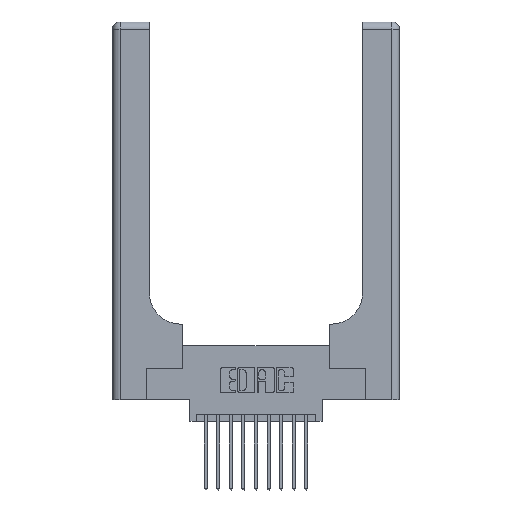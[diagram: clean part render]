
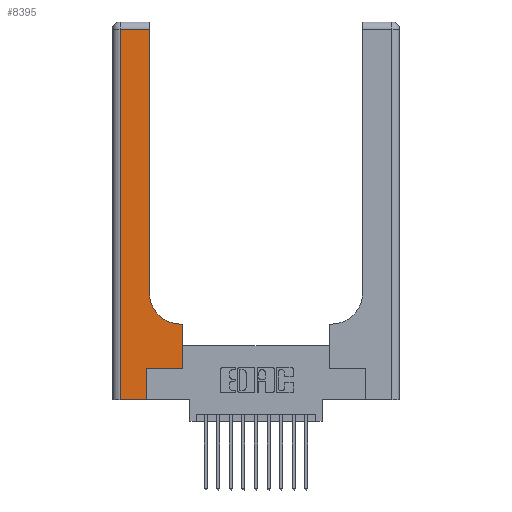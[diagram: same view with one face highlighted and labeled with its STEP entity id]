
A CAD part, top view. The second image highlights one B-rep face of the part: STEP entity #8395.
In plain terms, the highlighted planar face has unit normal (0, 0, 1).
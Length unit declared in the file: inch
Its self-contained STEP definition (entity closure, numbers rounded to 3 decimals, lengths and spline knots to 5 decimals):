
#37 = DIRECTION ( 'NONE',  ( 1., 0., 0. ) ) ;
#104 = VECTOR ( 'NONE', #10363, 39.37008 ) ;
#362 = LINE ( 'NONE', #11340, #13898 ) ;
#521 = LINE ( 'NONE', #15537, #104 ) ;
#1140 = CARTESIAN_POINT ( 'NONE',  ( 0.5585, 0.25, 0.37 ) ) ;
#1219 = VERTEX_POINT ( 'NONE', #10721 ) ;
#1307 = VERTEX_POINT ( 'NONE', #4497 ) ;
#1602 = LINE ( 'NONE', #8688, #14653 ) ;
#1817 = CIRCLE ( 'NONE', #6236, 0.25 ) ;
#2074 = CARTESIAN_POINT ( 'NONE',  ( 0.269, 0., 0.37 ) ) ;
#2140 = ORIENTED_EDGE ( 'NONE', *, *, #8368, .T. ) ;
#2536 = EDGE_CURVE ( 'NONE', #1307, #12621, #1602, .T. ) ;
#2644 = LINE ( 'NONE', #6530, #9198 ) ;
#2702 = VERTEX_POINT ( 'NONE', #1140 ) ;
#2889 = EDGE_CURVE ( 'NONE', #15873, #1219, #1817, .T. ) ;
#3220 = EDGE_CURVE ( 'NONE', #14287, #15873, #13449, .T. ) ;
#3399 = EDGE_CURVE ( 'NONE', #1219, #1307, #521, .T. ) ;
#3471 = DIRECTION ( 'NONE',  ( -1., 0., 0. ) ) ;
#3485 = FACE_OUTER_BOUND ( 'NONE', #14809, .T. ) ;
#4211 = ORIENTED_EDGE ( 'NONE', *, *, #3399, .T. ) ;
#4497 = CARTESIAN_POINT ( 'NONE',  ( 0.2915, 2.94, 0.37 ) ) ;
#4805 = DIRECTION ( 'NONE',  ( 0., 1., 0. ) ) ;
#4854 = DIRECTION ( 'NONE',  ( -1., 0., 0. ) ) ;
#4859 = PLANE ( 'NONE',  #8008 ) ;
#4885 = ORIENTED_EDGE ( 'NONE', *, *, #3220, .T. ) ;
#5260 = ORIENTED_EDGE ( 'NONE', *, *, #5963, .T. ) ;
#5262 = CARTESIAN_POINT ( 'NONE',  ( 0.269, 0.25, 0.37 ) ) ;
#5963 = EDGE_CURVE ( 'NONE', #10393, #14970, #16134, .T. ) ;
#6160 = DIRECTION ( 'NONE',  ( -1., 0., 0. ) ) ;
#6236 = AXIS2_PLACEMENT_3D ( 'NONE', #14668, #6862, #15933 ) ;
#6530 = CARTESIAN_POINT ( 'NONE',  ( 0.269, 0.25, 0.37 ) ) ;
#6651 = EDGE_CURVE ( 'NONE', #9863, #10393, #13339, .T. ) ;
#6862 = DIRECTION ( 'NONE',  ( 0., 0., -1. ) ) ;
#6885 = DIRECTION ( 'NONE',  ( 1., 0., 0. ) ) ;
#7643 = VECTOR ( 'NONE', #6885, 39.37008 ) ;
#7901 = DIRECTION ( 'NONE',  ( 0., -1., 0. ) ) ;
#8008 = AXIS2_PLACEMENT_3D ( 'NONE', #12649, #13997, #6160 ) ;
#8184 = CARTESIAN_POINT ( 'NONE',  ( 0.06, 2.94, 0.37 ) ) ;
#8368 = EDGE_CURVE ( 'NONE', #2702, #14287, #362, .T. ) ;
#8395 = ADVANCED_FACE ( 'NONE', ( #3485 ), #4859, .F. ) ;
#8688 = CARTESIAN_POINT ( 'NONE',  ( 0., 2.94, 0.37 ) ) ;
#9198 = VECTOR ( 'NONE', #37, 39.37008 ) ;
#9303 = VECTOR ( 'NONE', #13883, 39.37008 ) ;
#9345 = CARTESIAN_POINT ( 'NONE',  ( 0.269, 0., 0.37 ) ) ;
#9600 = VECTOR ( 'NONE', #4854, 39.37008 ) ;
#9863 = VERTEX_POINT ( 'NONE', #10834 ) ;
#10087 = CARTESIAN_POINT ( 'NONE',  ( 0.2915, 0.6, 0.37 ) ) ;
#10334 = EDGE_CURVE ( 'NONE', #12621, #9863, #14892, .T. ) ;
#10363 = DIRECTION ( 'NONE',  ( 0., 1., 0. ) ) ;
#10393 = VERTEX_POINT ( 'NONE', #9345 ) ;
#10721 = CARTESIAN_POINT ( 'NONE',  ( 0.2915, 0.85, 0.37 ) ) ;
#10834 = CARTESIAN_POINT ( 'NONE',  ( 0.06, 0., 0.37 ) ) ;
#10854 = ORIENTED_EDGE ( 'NONE', *, *, #10334, .T. ) ;
#11127 = EDGE_CURVE ( 'NONE', #14970, #2702, #2644, .T. ) ;
#11340 = CARTESIAN_POINT ( 'NONE',  ( 0.5585, 0.25, 0.37 ) ) ;
#12313 = ORIENTED_EDGE ( 'NONE', *, *, #6651, .T. ) ;
#12621 = VERTEX_POINT ( 'NONE', #8184 ) ;
#12649 = CARTESIAN_POINT ( 'NONE',  ( 0., 3., 0.37 ) ) ;
#12746 = CARTESIAN_POINT ( 'NONE',  ( 0.5415, 0.6, 0.37 ) ) ;
#13014 = CARTESIAN_POINT ( 'NONE',  ( 0.5585, 0.6, 0.37 ) ) ;
#13339 = LINE ( 'NONE', #14693, #7643 ) ;
#13449 = LINE ( 'NONE', #10087, #9600 ) ;
#13556 = ORIENTED_EDGE ( 'NONE', *, *, #2889, .T. ) ;
#13883 = DIRECTION ( 'NONE',  ( 0., 1., 0. ) ) ;
#13898 = VECTOR ( 'NONE', #4805, 39.37008 ) ;
#13997 = DIRECTION ( 'NONE',  ( 0., 0., -1. ) ) ;
#14095 = VECTOR ( 'NONE', #7901, 39.37008 ) ;
#14287 = VERTEX_POINT ( 'NONE', #13014 ) ;
#14653 = VECTOR ( 'NONE', #3471, 39.37008 ) ;
#14668 = CARTESIAN_POINT ( 'NONE',  ( 0.5415, 0.85, 0.37 ) ) ;
#14693 = CARTESIAN_POINT ( 'NONE',  ( 0., 0., 0.37 ) ) ;
#14809 = EDGE_LOOP ( 'NONE', ( #4211, #16591, #10854, #12313, #5260, #16488, #2140, #4885, #13556 ) ) ;
#14892 = LINE ( 'NONE', #15656, #14095 ) ;
#14970 = VERTEX_POINT ( 'NONE', #5262 ) ;
#15537 = CARTESIAN_POINT ( 'NONE',  ( 0.2915, 3., 0.37 ) ) ;
#15656 = CARTESIAN_POINT ( 'NONE',  ( 0.06, 3., 0.37 ) ) ;
#15873 = VERTEX_POINT ( 'NONE', #12746 ) ;
#15933 = DIRECTION ( 'NONE',  ( 1., 0., 0. ) ) ;
#16134 = LINE ( 'NONE', #2074, #9303 ) ;
#16488 = ORIENTED_EDGE ( 'NONE', *, *, #11127, .T. ) ;
#16591 = ORIENTED_EDGE ( 'NONE', *, *, #2536, .T. ) ;
